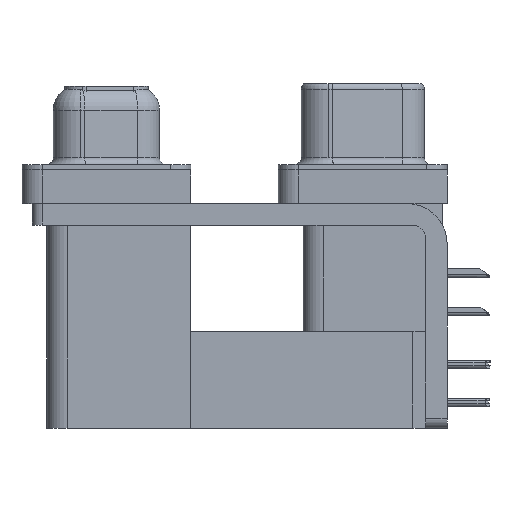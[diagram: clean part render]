
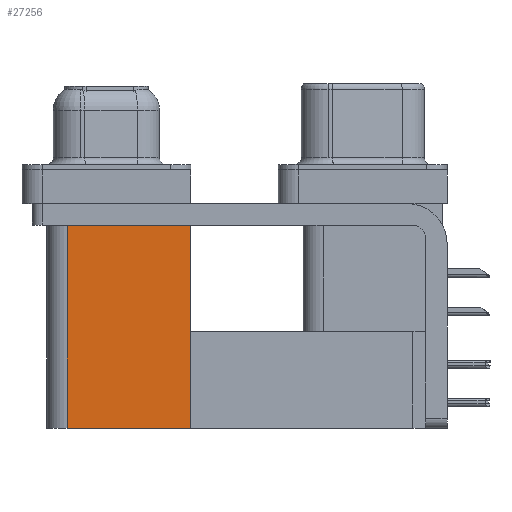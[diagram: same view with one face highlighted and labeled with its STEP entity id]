
A CAD part, left-side view. The second image highlights one B-rep face of the part: STEP entity #27256.
In plain terms, the highlighted planar face has unit normal (-1, 0, 0).
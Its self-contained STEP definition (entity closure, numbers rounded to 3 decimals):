
#868 = VERTEX_POINT ( 'NONE', #7818 ) ;
#1829 = CARTESIAN_POINT ( 'NONE',  ( 3.765, 12.775, -19.2 ) ) ;
#3528 = DIRECTION ( 'NONE',  ( 0., 1., 0. ) ) ;
#5746 = VECTOR ( 'NONE', #32279, 1000. ) ;
#5852 = VERTEX_POINT ( 'NONE', #10075 ) ;
#6280 = ORIENTED_EDGE ( 'NONE', *, *, #28785, .T. ) ;
#6424 = EDGE_CURVE ( 'NONE', #5852, #22867, #30529, .T. ) ;
#6639 = LINE ( 'NONE', #19463, #5746 ) ;
#6643 = EDGE_LOOP ( 'NONE', ( #31155, #36594, #23131, #6280 ) ) ;
#7818 = CARTESIAN_POINT ( 'NONE',  ( 3.765, 12.775, -2.5 ) ) ;
#9438 = LINE ( 'NONE', #22267, #27806 ) ;
#10075 = CARTESIAN_POINT ( 'NONE',  ( 3.765, 12.775, -19.2 ) ) ;
#10854 = VECTOR ( 'NONE', #15262, 1000. ) ;
#11952 = DIRECTION ( 'NONE',  ( 1., 0., 0. ) ) ;
#12350 = VECTOR ( 'NONE', #17470, 1000. ) ;
#14888 = EDGE_CURVE ( 'NONE', #22867, #18246, #6639, .T. ) ;
#15262 = DIRECTION ( 'NONE',  ( 0., 0., 1. ) ) ;
#17470 = DIRECTION ( 'NONE',  ( 0., 1., 0. ) ) ;
#18246 = VERTEX_POINT ( 'NONE', #25632 ) ;
#19463 = CARTESIAN_POINT ( 'NONE',  ( 3.765, 21.975, -19.2 ) ) ;
#22267 = CARTESIAN_POINT ( 'NONE',  ( 3.765, 12.775, -2.5 ) ) ;
#22867 = VERTEX_POINT ( 'NONE', #29749 ) ;
#23131 = ORIENTED_EDGE ( 'NONE', *, *, #6424, .F. ) ;
#25183 = DIRECTION ( 'NONE',  ( 0., 1., 0. ) ) ;
#25632 = CARTESIAN_POINT ( 'NONE',  ( 3.765, 21.975, -2.5 ) ) ;
#26942 = CARTESIAN_POINT ( 'NONE',  ( 3.765, 12.775, -19.2 ) ) ;
#27256 = ADVANCED_FACE ( 'NONE', ( #40336 ), #37812, .F. ) ;
#27290 = LINE ( 'NONE', #1829, #10854 ) ;
#27806 = VECTOR ( 'NONE', #3528, 1000. ) ;
#28785 = EDGE_CURVE ( 'NONE', #5852, #868, #27290, .T. ) ;
#29749 = CARTESIAN_POINT ( 'NONE',  ( 3.765, 21.975, -19.2 ) ) ;
#30529 = LINE ( 'NONE', #26942, #12350 ) ;
#31155 = ORIENTED_EDGE ( 'NONE', *, *, #38691, .T. ) ;
#31498 = CARTESIAN_POINT ( 'NONE',  ( 3.765, 12.775, -19.2 ) ) ;
#32279 = DIRECTION ( 'NONE',  ( 0., 0., 1. ) ) ;
#36594 = ORIENTED_EDGE ( 'NONE', *, *, #14888, .F. ) ;
#37812 = PLANE ( 'NONE',  #40939 ) ;
#38691 = EDGE_CURVE ( 'NONE', #868, #18246, #9438, .T. ) ;
#40336 = FACE_OUTER_BOUND ( 'NONE', #6643, .T. ) ;
#40939 = AXIS2_PLACEMENT_3D ( 'NONE', #31498, #11952, #25183 ) ;
